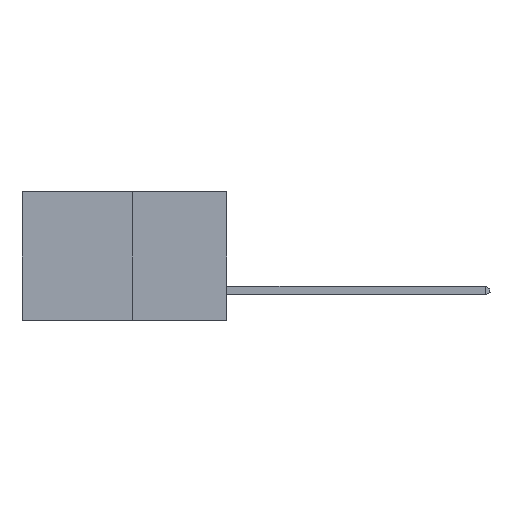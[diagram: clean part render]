
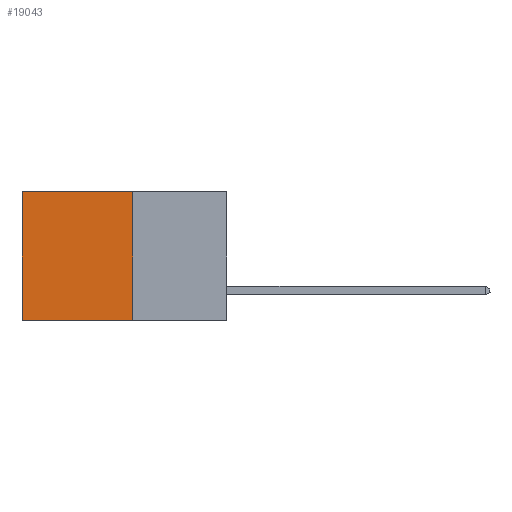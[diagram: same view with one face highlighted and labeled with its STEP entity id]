
A CAD part, left-side view. The second image highlights one B-rep face of the part: STEP entity #19043.
In plain terms, the highlighted planar face has unit normal (-1, 0, 0).
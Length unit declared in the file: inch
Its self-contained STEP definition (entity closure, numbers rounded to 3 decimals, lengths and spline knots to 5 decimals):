
#311 = LINE ( 'NONE', #14152, #17700 ) ;
#842 = VERTEX_POINT ( 'NONE', #19360 ) ;
#1529 = VECTOR ( 'NONE', #15491, 39.37008 ) ;
#1543 = VECTOR ( 'NONE', #11675, 39.37008 ) ;
#2085 = LINE ( 'NONE', #9987, #1543 ) ;
#3493 = FACE_OUTER_BOUND ( 'NONE', #9572, .T. ) ;
#4118 = AXIS2_PLACEMENT_3D ( 'NONE', #6563, #18140, #8199 ) ;
#6176 = DIRECTION ( 'NONE',  ( 0., 1., 0. ) ) ;
#6563 = CARTESIAN_POINT ( 'NONE',  ( 0.277, 0.27, -0.37 ) ) ;
#7606 = ORIENTED_EDGE ( 'NONE', *, *, #8383, .F. ) ;
#8199 = DIRECTION ( 'NONE',  ( 0., 0., -1. ) ) ;
#8216 = VECTOR ( 'NONE', #6176, 39.37008 ) ;
#8383 = EDGE_CURVE ( 'NONE', #20350, #15013, #14969, .T. ) ;
#8717 = LINE ( 'NONE', #19439, #8216 ) ;
#9572 = EDGE_LOOP ( 'NONE', ( #13723, #11326, #7606, #15428 ) ) ;
#9987 = CARTESIAN_POINT ( 'NONE',  ( 0.277, 0.27, 0. ) ) ;
#11220 = VERTEX_POINT ( 'NONE', #11592 ) ;
#11326 = ORIENTED_EDGE ( 'NONE', *, *, #19672, .F. ) ;
#11592 = CARTESIAN_POINT ( 'NONE',  ( 0.277, 0.59, 0. ) ) ;
#11675 = DIRECTION ( 'NONE',  ( 0., 1., 0. ) ) ;
#13723 = ORIENTED_EDGE ( 'NONE', *, *, #20119, .T. ) ;
#14152 = CARTESIAN_POINT ( 'NONE',  ( 0.277, 0.59, -0.37 ) ) ;
#14230 = DIRECTION ( 'NONE',  ( 0., 0., -1. ) ) ;
#14969 = LINE ( 'NONE', #17151, #1529 ) ;
#15013 = VERTEX_POINT ( 'NONE', #15761 ) ;
#15428 = ORIENTED_EDGE ( 'NONE', *, *, #19748, .T. ) ;
#15491 = DIRECTION ( 'NONE',  ( 0., 0., -1. ) ) ;
#15761 = CARTESIAN_POINT ( 'NONE',  ( 0.277, 0.27, -0.37 ) ) ;
#17151 = CARTESIAN_POINT ( 'NONE',  ( 0.277, 0.27, -0.37 ) ) ;
#17700 = VECTOR ( 'NONE', #14230, 39.37008 ) ;
#18140 = DIRECTION ( 'NONE',  ( 1., 0., 0. ) ) ;
#19043 = ADVANCED_FACE ( 'NONE', ( #3493 ), #21388, .F. ) ;
#19360 = CARTESIAN_POINT ( 'NONE',  ( 0.277, 0.59, -0.37 ) ) ;
#19439 = CARTESIAN_POINT ( 'NONE',  ( 0.277, 0.27, -0.37 ) ) ;
#19672 = EDGE_CURVE ( 'NONE', #15013, #842, #8717, .T. ) ;
#19748 = EDGE_CURVE ( 'NONE', #20350, #11220, #2085, .T. ) ;
#19777 = CARTESIAN_POINT ( 'NONE',  ( 0.277, 0.27, 0. ) ) ;
#20119 = EDGE_CURVE ( 'NONE', #11220, #842, #311, .T. ) ;
#20350 = VERTEX_POINT ( 'NONE', #19777 ) ;
#21388 = PLANE ( 'NONE',  #4118 ) ;
